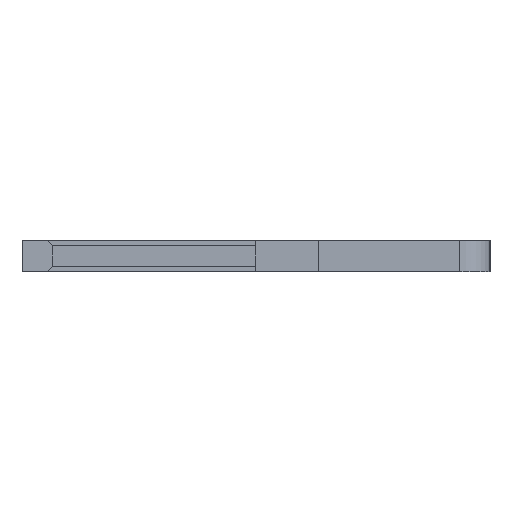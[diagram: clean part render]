
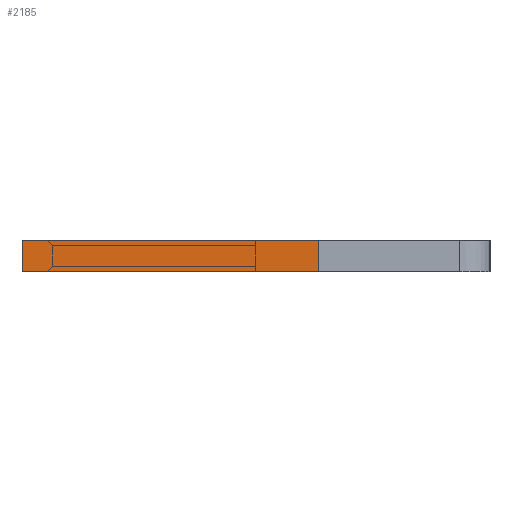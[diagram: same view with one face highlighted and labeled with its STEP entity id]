
A CAD part, left-side view. The second image highlights one B-rep face of the part: STEP entity #2185.
In plain terms, the highlighted face is planar.
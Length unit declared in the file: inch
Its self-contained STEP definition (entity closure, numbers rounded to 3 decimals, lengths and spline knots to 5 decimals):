
#59 = CARTESIAN_POINT ( 'NONE',  ( 0.01, -0.04, -0.04 ) ) ;
#107 = FACE_OUTER_BOUND ( 'NONE', #2277, .T. ) ;
#153 = VERTEX_POINT ( 'NONE', #2302 ) ;
#363 = VECTOR ( 'NONE', #1355, 39.37008 ) ;
#433 = CARTESIAN_POINT ( 'NONE',  ( 0.01, 0.15, -0.04 ) ) ;
#454 = PLANE ( 'NONE',  #679 ) ;
#654 = ORIENTED_EDGE ( 'NONE', *, *, #2087, .F. ) ;
#679 = AXIS2_PLACEMENT_3D ( 'NONE', #1744, #1726, #1203 ) ;
#706 = LINE ( 'NONE', #433, #1084 ) ;
#766 = VECTOR ( 'NONE', #1611, 39.37008 ) ;
#774 = VERTEX_POINT ( 'NONE', #1449 ) ;
#796 = LINE ( 'NONE', #1420, #766 ) ;
#856 = LINE ( 'NONE', #1108, #2098 ) ;
#903 = EDGE_CURVE ( 'NONE', #1247, #774, #796, .T. ) ;
#1084 = VECTOR ( 'NONE', #1557, 39.37008 ) ;
#1108 = CARTESIAN_POINT ( 'NONE',  ( -0.01, 0.15, -0.04 ) ) ;
#1123 = CARTESIAN_POINT ( 'NONE',  ( 0.01, -0.04, -0.04 ) ) ;
#1203 = DIRECTION ( 'NONE',  ( 1., 0., 0. ) ) ;
#1239 = ORIENTED_EDGE ( 'NONE', *, *, #1347, .T. ) ;
#1247 = VERTEX_POINT ( 'NONE', #1123 ) ;
#1287 = ORIENTED_EDGE ( 'NONE', *, *, #903, .F. ) ;
#1347 = EDGE_CURVE ( 'NONE', #2245, #153, #856, .T. ) ;
#1355 = DIRECTION ( 'NONE',  ( -1., 0., 0. ) ) ;
#1420 = CARTESIAN_POINT ( 'NONE',  ( 0.01, 0.15, -0.04 ) ) ;
#1449 = CARTESIAN_POINT ( 'NONE',  ( 0.01, 0.15, -0.04 ) ) ;
#1557 = DIRECTION ( 'NONE',  ( -1., 0., 0. ) ) ;
#1611 = DIRECTION ( 'NONE',  ( 0., 1., 0. ) ) ;
#1717 = LINE ( 'NONE', #59, #363 ) ;
#1726 = DIRECTION ( 'NONE',  ( 0., 0., 1. ) ) ;
#1744 = CARTESIAN_POINT ( 'NONE',  ( 0.01, 0.15, -0.04 ) ) ;
#1940 = EDGE_CURVE ( 'NONE', #1247, #2245, #1717, .T. ) ;
#2087 = EDGE_CURVE ( 'NONE', #774, #153, #706, .T. ) ;
#2098 = VECTOR ( 'NONE', #2219, 39.37008 ) ;
#2156 = ORIENTED_EDGE ( 'NONE', *, *, #1940, .T. ) ;
#2185 = ADVANCED_FACE ( 'NONE', ( #107 ), #454, .F. ) ;
#2219 = DIRECTION ( 'NONE',  ( 0., 1., 0. ) ) ;
#2245 = VERTEX_POINT ( 'NONE', #2295 ) ;
#2277 = EDGE_LOOP ( 'NONE', ( #1239, #654, #1287, #2156 ) ) ;
#2295 = CARTESIAN_POINT ( 'NONE',  ( -0.01, -0.04, -0.04 ) ) ;
#2302 = CARTESIAN_POINT ( 'NONE',  ( -0.01, 0.15, -0.04 ) ) ;
